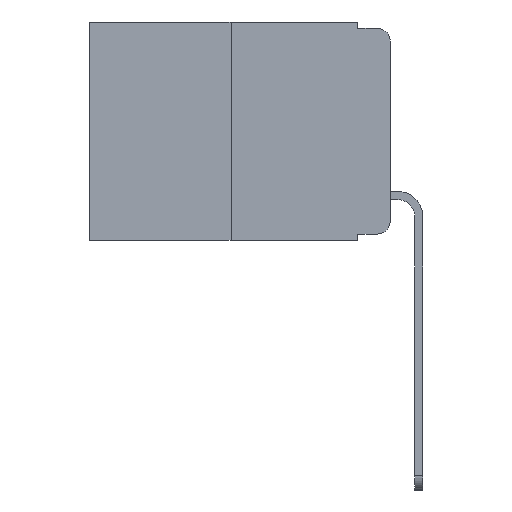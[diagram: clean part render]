
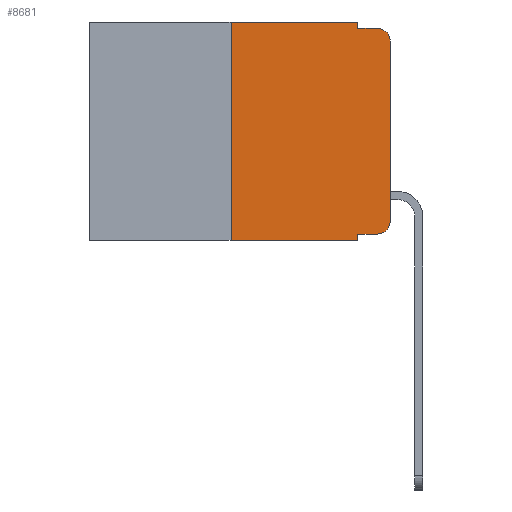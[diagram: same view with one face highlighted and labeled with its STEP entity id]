
A CAD part, left-side view. The second image highlights one B-rep face of the part: STEP entity #8681.
In plain terms, the highlighted planar face has unit normal (-1, 0, 0).
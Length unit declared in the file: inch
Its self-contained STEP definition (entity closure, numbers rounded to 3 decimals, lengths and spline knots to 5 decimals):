
#625 = AXIS2_PLACEMENT_3D ( 'NONE', #3327, #14059, #7323 ) ;
#680 = CARTESIAN_POINT ( 'NONE',  ( 0., 0.25, -0.343 ) ) ;
#856 = EDGE_CURVE ( 'NONE', #8220, #7221, #10390, .T. ) ;
#1120 = AXIS2_PLACEMENT_3D ( 'NONE', #3906, #4011, #2717 ) ;
#1306 = EDGE_CURVE ( 'NONE', #15814, #8220, #3209, .T. ) ;
#1426 = VERTEX_POINT ( 'NONE', #10107 ) ;
#1630 = CIRCLE ( 'NONE', #1120, 0.02 ) ;
#1720 = CARTESIAN_POINT ( 'NONE',  ( 0., 0.25, 0. ) ) ;
#2039 = ORIENTED_EDGE ( 'NONE', *, *, #1306, .T. ) ;
#2154 = EDGE_CURVE ( 'NONE', #11220, #15814, #16738, .T. ) ;
#2228 = VECTOR ( 'NONE', #3555, 39.37008 ) ;
#2717 = DIRECTION ( 'NONE',  ( 0., 0., -1. ) ) ;
#2725 = DIRECTION ( 'NONE',  ( 0., 0., -1. ) ) ;
#2876 = ORIENTED_EDGE ( 'NONE', *, *, #3409, .F. ) ;
#3209 = CIRCLE ( 'NONE', #625, 0.02 ) ;
#3327 = CARTESIAN_POINT ( 'NONE',  ( 0., 0.02, -0.313 ) ) ;
#3409 = EDGE_CURVE ( 'NONE', #6211, #16789, #4013, .T. ) ;
#3496 = CARTESIAN_POINT ( 'NONE',  ( 0., 0.473, 0. ) ) ;
#3555 = DIRECTION ( 'NONE',  ( 0., -1., 0. ) ) ;
#3906 = CARTESIAN_POINT ( 'NONE',  ( 0., 0.02, -0.03 ) ) ;
#4011 = DIRECTION ( 'NONE',  ( -1., 0., 0. ) ) ;
#4013 = LINE ( 'NONE', #6772, #9906 ) ;
#4540 = DIRECTION ( 'NONE',  ( 0., 0., -1. ) ) ;
#4937 = CARTESIAN_POINT ( 'NONE',  ( 0., 0.473, -0.343 ) ) ;
#5034 = EDGE_CURVE ( 'NONE', #7221, #16789, #1630, .T. ) ;
#5074 = CARTESIAN_POINT ( 'NONE',  ( 0., 0.051, -0.01 ) ) ;
#5298 = ORIENTED_EDGE ( 'NONE', *, *, #10211, .F. ) ;
#5726 = DIRECTION ( 'NONE',  ( 0., 0., -1. ) ) ;
#5805 = VERTEX_POINT ( 'NONE', #12140 ) ;
#6047 = CARTESIAN_POINT ( 'NONE',  ( 0., 0., 0. ) ) ;
#6211 = VERTEX_POINT ( 'NONE', #5074 ) ;
#6517 = VECTOR ( 'NONE', #15165, 39.37008 ) ;
#6772 = CARTESIAN_POINT ( 'NONE',  ( 0., 0.051, -0.01 ) ) ;
#7221 = VERTEX_POINT ( 'NONE', #7762 ) ;
#7308 = CARTESIAN_POINT ( 'NONE',  ( 0., 0.02, -0.01 ) ) ;
#7323 = DIRECTION ( 'NONE',  ( 0., 0., -1. ) ) ;
#7568 = VERTEX_POINT ( 'NONE', #16889 ) ;
#7571 = EDGE_CURVE ( 'NONE', #10274, #1426, #8292, .T. ) ;
#7699 = CARTESIAN_POINT ( 'NONE',  ( 0., 0., -0.313 ) ) ;
#7762 = CARTESIAN_POINT ( 'NONE',  ( 0., 0., -0.03 ) ) ;
#8220 = VERTEX_POINT ( 'NONE', #7699 ) ;
#8292 = LINE ( 'NONE', #4937, #15693 ) ;
#8513 = DIRECTION ( 'NONE',  ( 1., 0., 0. ) ) ;
#8681 = ADVANCED_FACE ( 'NONE', ( #17345 ), #12438, .F. ) ;
#8704 = DIRECTION ( 'NONE',  ( 0., 0., 1. ) ) ;
#9133 = CARTESIAN_POINT ( 'NONE',  ( 0., 0.02, -0.333 ) ) ;
#9145 = VECTOR ( 'NONE', #8704, 39.37008 ) ;
#9461 = CARTESIAN_POINT ( 'NONE',  ( 0., 0.051, -0.333 ) ) ;
#9493 = EDGE_LOOP ( 'NONE', ( #12028, #13740, #2876, #14168, #15191, #5298, #16452, #16535, #15132, #2039 ) ) ;
#9906 = VECTOR ( 'NONE', #16458, 39.37008 ) ;
#10107 = CARTESIAN_POINT ( 'NONE',  ( 0., 0.051, -0.343 ) ) ;
#10211 = EDGE_CURVE ( 'NONE', #10274, #5805, #13042, .T. ) ;
#10274 = VERTEX_POINT ( 'NONE', #680 ) ;
#10390 = LINE ( 'NONE', #6047, #9145 ) ;
#10674 = VECTOR ( 'NONE', #2725, 39.37008 ) ;
#10780 = CARTESIAN_POINT ( 'NONE',  ( 0., 0.051, 0. ) ) ;
#11086 = LINE ( 'NONE', #10780, #10674 ) ;
#11139 = CARTESIAN_POINT ( 'NONE',  ( 0., 0.473, 0. ) ) ;
#11184 = CARTESIAN_POINT ( 'NONE',  ( 0., 0.051, 0. ) ) ;
#11220 = VERTEX_POINT ( 'NONE', #9461 ) ;
#11279 = EDGE_CURVE ( 'NONE', #7568, #6211, #11086, .T. ) ;
#11793 = VECTOR ( 'NONE', #4540, 39.37008 ) ;
#12028 = ORIENTED_EDGE ( 'NONE', *, *, #856, .T. ) ;
#12140 = CARTESIAN_POINT ( 'NONE',  ( 0., 0.25, 0. ) ) ;
#12438 = PLANE ( 'NONE',  #17242 ) ;
#12451 = EDGE_CURVE ( 'NONE', #5805, #7568, #16373, .T. ) ;
#13042 = LINE ( 'NONE', #1720, #6517 ) ;
#13740 = ORIENTED_EDGE ( 'NONE', *, *, #5034, .T. ) ;
#14059 = DIRECTION ( 'NONE',  ( -1., 0., 0. ) ) ;
#14168 = ORIENTED_EDGE ( 'NONE', *, *, #11279, .F. ) ;
#14656 = EDGE_CURVE ( 'NONE', #11220, #1426, #15854, .T. ) ;
#15026 = VECTOR ( 'NONE', #15880, 39.37008 ) ;
#15132 = ORIENTED_EDGE ( 'NONE', *, *, #2154, .T. ) ;
#15165 = DIRECTION ( 'NONE',  ( 0., 0., 1. ) ) ;
#15191 = ORIENTED_EDGE ( 'NONE', *, *, #12451, .F. ) ;
#15583 = DIRECTION ( 'NONE',  ( 0., -1., 0. ) ) ;
#15646 = CARTESIAN_POINT ( 'NONE',  ( 0., 0.051, -0.333 ) ) ;
#15693 = VECTOR ( 'NONE', #15583, 39.37008 ) ;
#15814 = VERTEX_POINT ( 'NONE', #9133 ) ;
#15854 = LINE ( 'NONE', #11184, #11793 ) ;
#15880 = DIRECTION ( 'NONE',  ( 0., -1., 0. ) ) ;
#16373 = LINE ( 'NONE', #3496, #2228 ) ;
#16452 = ORIENTED_EDGE ( 'NONE', *, *, #7571, .T. ) ;
#16458 = DIRECTION ( 'NONE',  ( 0., -1., 0. ) ) ;
#16535 = ORIENTED_EDGE ( 'NONE', *, *, #14656, .F. ) ;
#16738 = LINE ( 'NONE', #15646, #15026 ) ;
#16789 = VERTEX_POINT ( 'NONE', #7308 ) ;
#16889 = CARTESIAN_POINT ( 'NONE',  ( 0., 0.051, 0. ) ) ;
#17242 = AXIS2_PLACEMENT_3D ( 'NONE', #11139, #8513, #5726 ) ;
#17345 = FACE_OUTER_BOUND ( 'NONE', #9493, .T. ) ;
